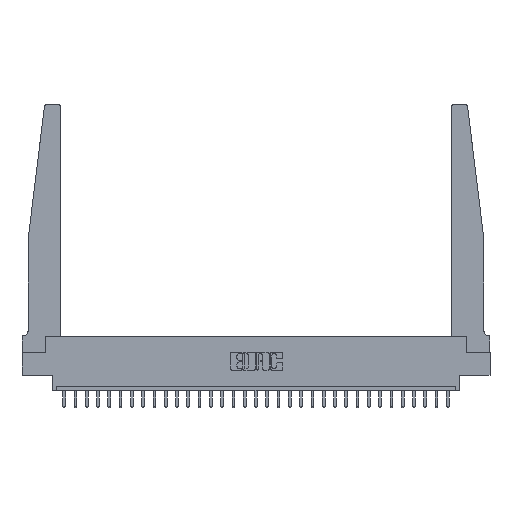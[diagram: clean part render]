
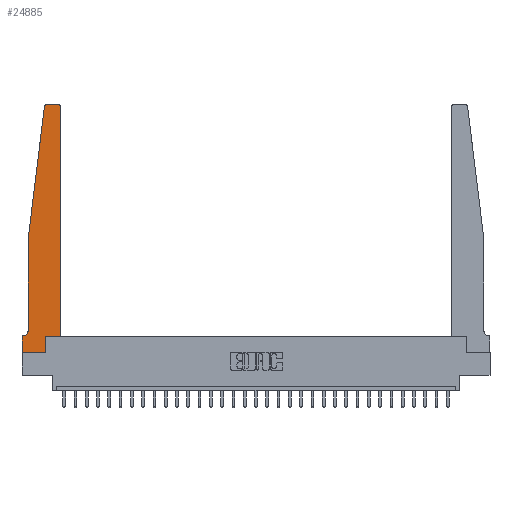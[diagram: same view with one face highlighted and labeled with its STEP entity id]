
A CAD part, top view. The second image highlights one B-rep face of the part: STEP entity #24885.
In plain terms, the highlighted planar face has unit normal (0, 0, 1).
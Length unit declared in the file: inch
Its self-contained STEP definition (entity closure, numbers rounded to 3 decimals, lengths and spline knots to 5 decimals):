
#10 = CARTESIAN_POINT ( 'NONE',  ( 0.24675, 2.72367, 0.37 ) ) ;
#73 = CARTESIAN_POINT ( 'NONE',  ( 0., 0., 0.37 ) ) ;
#170 = VERTEX_POINT ( 'NONE', #11695 ) ;
#612 = EDGE_CURVE ( 'NONE', #23524, #14252, #2229, .T. ) ;
#1268 = DIRECTION ( 'NONE',  ( -1., 0., 0. ) ) ;
#1519 = DIRECTION ( 'NONE',  ( 1., 0., 0. ) ) ;
#1872 = LINE ( 'NONE', #5742, #25076 ) ;
#1993 = EDGE_CURVE ( 'NONE', #12487, #2360, #16868, .T. ) ;
#2229 = CIRCLE ( 'NONE', #15833, 0.05 ) ;
#2281 = VERTEX_POINT ( 'NONE', #26075 ) ;
#2325 = VECTOR ( 'NONE', #8827, 39.37008 ) ;
#2360 = VERTEX_POINT ( 'NONE', #24345 ) ;
#2858 = VERTEX_POINT ( 'NONE', #25354 ) ;
#3524 = LINE ( 'NONE', #16733, #23945 ) ;
#3968 = FACE_OUTER_BOUND ( 'NONE', #18637, .T. ) ;
#4236 = CARTESIAN_POINT ( 'NONE',  ( 0., 0.1875, 0.37 ) ) ;
#4372 = LINE ( 'NONE', #73, #8648 ) ;
#5339 = LINE ( 'NONE', #15696, #6219 ) ;
#5365 = DIRECTION ( 'NONE',  ( -1., 0., 0. ) ) ;
#5742 = CARTESIAN_POINT ( 'NONE',  ( 0.065, 1.25, 0.37 ) ) ;
#6091 = DIRECTION ( 'NONE',  ( 0., 1., 0. ) ) ;
#6106 = DIRECTION ( 'NONE',  ( 0., 0., 1. ) ) ;
#6219 = VECTOR ( 'NONE', #11407, 39.37008 ) ;
#6237 = DIRECTION ( 'NONE',  ( 0., -1., 0. ) ) ;
#6447 = LINE ( 'NONE', #21919, #2325 ) ;
#7388 = ORIENTED_EDGE ( 'NONE', *, *, #9396, .T. ) ;
#8284 = EDGE_CURVE ( 'NONE', #2281, #23524, #6447, .T. ) ;
#8383 = VERTEX_POINT ( 'NONE', #10 ) ;
#8648 = VECTOR ( 'NONE', #19579, 39.37008 ) ;
#8827 = DIRECTION ( 'NONE',  ( 0., -1., 0. ) ) ;
#9396 = EDGE_CURVE ( 'NONE', #8383, #2281, #1872, .T. ) ;
#9584 = ORIENTED_EDGE ( 'NONE', *, *, #16714, .T. ) ;
#9906 = AXIS2_PLACEMENT_3D ( 'NONE', #25160, #24578, #9911 ) ;
#9911 = DIRECTION ( 'NONE',  ( 1., 0., 0. ) ) ;
#10938 = ORIENTED_EDGE ( 'NONE', *, *, #8284, .T. ) ;
#11407 = DIRECTION ( 'NONE',  ( 1., 0., 0. ) ) ;
#11695 = CARTESIAN_POINT ( 'NONE',  ( 0.395, 2.75, 0.37 ) ) ;
#12184 = AXIS2_PLACEMENT_3D ( 'NONE', #26442, #15347, #15624 ) ;
#12208 = CARTESIAN_POINT ( 'NONE',  ( 0.015, 0.2375, 0.37 ) ) ;
#12443 = DIRECTION ( 'NONE',  ( 0., 1., 0. ) ) ;
#12487 = VERTEX_POINT ( 'NONE', #18209 ) ;
#13031 = VECTOR ( 'NONE', #6237, 39.37008 ) ;
#13098 = VECTOR ( 'NONE', #25134, 39.37008 ) ;
#13127 = ORIENTED_EDGE ( 'NONE', *, *, #26672, .T. ) ;
#13490 = ORIENTED_EDGE ( 'NONE', *, *, #17454, .T. ) ;
#14247 = ORIENTED_EDGE ( 'NONE', *, *, #19984, .T. ) ;
#14252 = VERTEX_POINT ( 'NONE', #14442 ) ;
#14442 = CARTESIAN_POINT ( 'NONE',  ( 0.015, 0.1875, 0.37 ) ) ;
#14486 = DIRECTION ( 'NONE',  ( 0., 0., -1. ) ) ;
#14580 = CARTESIAN_POINT ( 'NONE',  ( 0.27653, 2.75, 0.37 ) ) ;
#14594 = CARTESIAN_POINT ( 'NONE',  ( 0.065, 0.1875, 0.37 ) ) ;
#14733 = LINE ( 'NONE', #25701, #13031 ) ;
#15002 = PLANE ( 'NONE',  #20807 ) ;
#15347 = DIRECTION ( 'NONE',  ( 0., 0., 1. ) ) ;
#15581 = VERTEX_POINT ( 'NONE', #19238 ) ;
#15624 = DIRECTION ( 'NONE',  ( 1., 0., 0. ) ) ;
#15696 = CARTESIAN_POINT ( 'NONE',  ( 0.425, 0.18, 0.37 ) ) ;
#15833 = AXIS2_PLACEMENT_3D ( 'NONE', #12208, #14486, #1268 ) ;
#16230 = ORIENTED_EDGE ( 'NONE', *, *, #1993, .T. ) ;
#16714 = EDGE_CURVE ( 'NONE', #170, #22043, #20716, .T. ) ;
#16733 = CARTESIAN_POINT ( 'NONE',  ( 0.2605, 0.18, 0.37 ) ) ;
#16868 = LINE ( 'NONE', #25557, #21841 ) ;
#17422 = EDGE_CURVE ( 'NONE', #22043, #8383, #21769, .T. ) ;
#17454 = EDGE_CURVE ( 'NONE', #2360, #170, #25405, .T. ) ;
#18013 = ORIENTED_EDGE ( 'NONE', *, *, #24854, .T. ) ;
#18209 = CARTESIAN_POINT ( 'NONE',  ( 0.425, 0.18, 0.37 ) ) ;
#18637 = EDGE_LOOP ( 'NONE', ( #9584, #23659, #7388, #10938, #18929, #14247, #18013, #27988, #26227, #13127, #16230, #13490 ) ) ;
#18753 = LINE ( 'NONE', #14594, #13098 ) ;
#18929 = ORIENTED_EDGE ( 'NONE', *, *, #612, .T. ) ;
#19238 = CARTESIAN_POINT ( 'NONE',  ( 0., 0.1875, 0.37 ) ) ;
#19579 = DIRECTION ( 'NONE',  ( 1., 0., 0. ) ) ;
#19782 = CARTESIAN_POINT ( 'NONE',  ( 0.065, 0.2375, 0.37 ) ) ;
#19984 = EDGE_CURVE ( 'NONE', #14252, #15581, #18753, .T. ) ;
#20716 = LINE ( 'NONE', #22857, #24423 ) ;
#20807 = AXIS2_PLACEMENT_3D ( 'NONE', #4236, #6106, #1519 ) ;
#20949 = DIRECTION ( 'NONE',  ( -0.122, -0.992, 0. ) ) ;
#21244 = EDGE_CURVE ( 'NONE', #2858, #22104, #4372, .T. ) ;
#21610 = CARTESIAN_POINT ( 'NONE',  ( 0.2605, 0.18, 0.37 ) ) ;
#21769 = CIRCLE ( 'NONE', #12184, 0.03 ) ;
#21841 = VECTOR ( 'NONE', #6091, 39.37008 ) ;
#21919 = CARTESIAN_POINT ( 'NONE',  ( 0.065, 1.25, 0.37 ) ) ;
#22043 = VERTEX_POINT ( 'NONE', #14580 ) ;
#22104 = VERTEX_POINT ( 'NONE', #27963 ) ;
#22857 = CARTESIAN_POINT ( 'NONE',  ( 0.25, 2.75, 0.37 ) ) ;
#23524 = VERTEX_POINT ( 'NONE', #19782 ) ;
#23659 = ORIENTED_EDGE ( 'NONE', *, *, #17422, .T. ) ;
#23897 = VERTEX_POINT ( 'NONE', #21610 ) ;
#23945 = VECTOR ( 'NONE', #12443, 39.37008 ) ;
#24071 = EDGE_CURVE ( 'NONE', #22104, #23897, #3524, .T. ) ;
#24345 = CARTESIAN_POINT ( 'NONE',  ( 0.425, 2.72, 0.37 ) ) ;
#24423 = VECTOR ( 'NONE', #5365, 39.37008 ) ;
#24578 = DIRECTION ( 'NONE',  ( 0., 0., 1. ) ) ;
#24854 = EDGE_CURVE ( 'NONE', #15581, #2858, #14733, .T. ) ;
#24885 = ADVANCED_FACE ( 'NONE', ( #3968 ), #15002, .T. ) ;
#25076 = VECTOR ( 'NONE', #20949, 39.37008 ) ;
#25134 = DIRECTION ( 'NONE',  ( -1., 0., 0. ) ) ;
#25160 = CARTESIAN_POINT ( 'NONE',  ( 0.395, 2.72, 0.37 ) ) ;
#25354 = CARTESIAN_POINT ( 'NONE',  ( 0., 0., 0.37 ) ) ;
#25405 = CIRCLE ( 'NONE', #9906, 0.03 ) ;
#25557 = CARTESIAN_POINT ( 'NONE',  ( 0.425, 0.18, 0.37 ) ) ;
#25701 = CARTESIAN_POINT ( 'NONE',  ( 0., 0., 0.37 ) ) ;
#26075 = CARTESIAN_POINT ( 'NONE',  ( 0.065, 1.25, 0.37 ) ) ;
#26227 = ORIENTED_EDGE ( 'NONE', *, *, #24071, .T. ) ;
#26442 = CARTESIAN_POINT ( 'NONE',  ( 0.27653, 2.72, 0.37 ) ) ;
#26672 = EDGE_CURVE ( 'NONE', #23897, #12487, #5339, .T. ) ;
#27963 = CARTESIAN_POINT ( 'NONE',  ( 0.2605, 0., 0.37 ) ) ;
#27988 = ORIENTED_EDGE ( 'NONE', *, *, #21244, .T. ) ;
